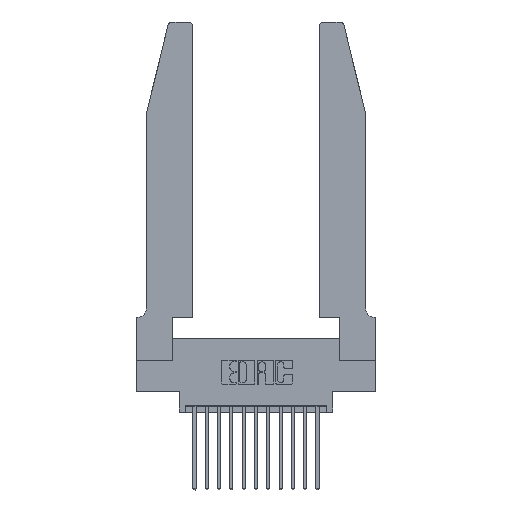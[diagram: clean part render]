
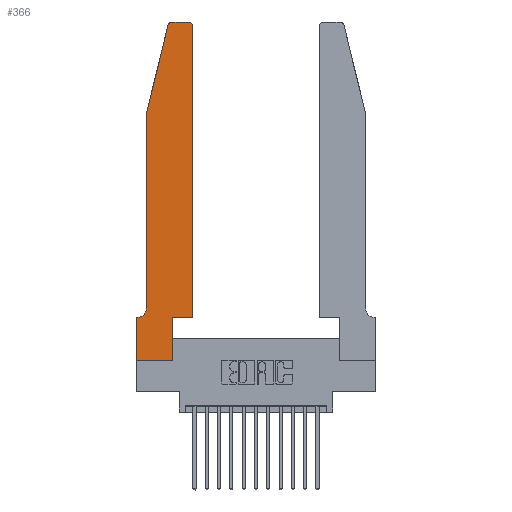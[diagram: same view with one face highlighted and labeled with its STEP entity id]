
A CAD part, top view. The second image highlights one B-rep face of the part: STEP entity #366.
In plain terms, the highlighted planar face has unit normal (0, 0, 1).
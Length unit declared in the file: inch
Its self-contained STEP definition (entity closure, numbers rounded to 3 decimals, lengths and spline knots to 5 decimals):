
#36 = DIRECTION ( 'NONE',  ( 1., 0., 0. ) ) ;
#366 = ADVANCED_FACE ( 'NONE', ( #13442 ), #1241, .T. ) ;
#414 = ORIENTED_EDGE ( 'NONE', *, *, #12444, .T. ) ;
#438 = LINE ( 'NONE', #11893, #1290 ) ;
#743 = EDGE_CURVE ( 'NONE', #1379, #2221, #4487, .T. ) ;
#882 = DIRECTION ( 'NONE',  ( 0., 0., -1. ) ) ;
#923 = CARTESIAN_POINT ( 'NONE',  ( 0.0055, 0.35, 0.37 ) ) ;
#1241 = PLANE ( 'NONE',  #9809 ) ;
#1269 = DIRECTION ( 'NONE',  ( 1., 0., 0. ) ) ;
#1290 = VECTOR ( 'NONE', #7604, 39.37008 ) ;
#1333 = CARTESIAN_POINT ( 'NONE',  ( 0.2865, 0.35, 0.37 ) ) ;
#1379 = VERTEX_POINT ( 'NONE', #923 ) ;
#1514 = VECTOR ( 'NONE', #6909, 39.37008 ) ;
#1750 = VECTOR ( 'NONE', #2633, 39.37008 ) ;
#1841 = VERTEX_POINT ( 'NONE', #9988 ) ;
#1915 = VECTOR ( 'NONE', #12813, 39.37008 ) ;
#2221 = VERTEX_POINT ( 'NONE', #14947 ) ;
#2362 = CARTESIAN_POINT ( 'NONE',  ( 0.2605, 2.75, 0.37 ) ) ;
#2605 = DIRECTION ( 'NONE',  ( 1., 0., 0. ) ) ;
#2621 = CARTESIAN_POINT ( 'NONE',  ( 0.2865, 0., 0.37 ) ) ;
#2633 = DIRECTION ( 'NONE',  ( 0., 1., 0. ) ) ;
#2759 = ORIENTED_EDGE ( 'NONE', *, *, #6326, .T. ) ;
#2988 = AXIS2_PLACEMENT_3D ( 'NONE', #9457, #16083, #1269 ) ;
#3045 = EDGE_CURVE ( 'NONE', #14107, #12969, #438, .T. ) ;
#3153 = DIRECTION ( 'NONE',  ( 0., -1., 0. ) ) ;
#3775 = VERTEX_POINT ( 'NONE', #7688 ) ;
#3949 = VERTEX_POINT ( 'NONE', #13862 ) ;
#4215 = CARTESIAN_POINT ( 'NONE',  ( 0.4205, 2.72, 0.37 ) ) ;
#4487 = LINE ( 'NONE', #15504, #1915 ) ;
#4493 = LINE ( 'NONE', #12278, #10693 ) ;
#4571 = VECTOR ( 'NONE', #3153, 39.37008 ) ;
#4719 = CARTESIAN_POINT ( 'NONE',  ( 0., 0., 0.37 ) ) ;
#5234 = DIRECTION ( 'NONE',  ( 1., 0., 0. ) ) ;
#5677 = LINE ( 'NONE', #2362, #12082 ) ;
#5840 = ORIENTED_EDGE ( 'NONE', *, *, #16171, .T. ) ;
#6107 = DIRECTION ( 'NONE',  ( 1., 0., 0. ) ) ;
#6326 = EDGE_CURVE ( 'NONE', #3775, #12021, #15503, .T. ) ;
#6420 = CARTESIAN_POINT ( 'NONE',  ( 0.0755, 0.42, 0.37 ) ) ;
#6518 = EDGE_LOOP ( 'NONE', ( #13067, #2759, #12171, #9908, #8247, #12234, #15975, #414, #17233, #5840, #12207, #11344 ) ) ;
#6736 = DIRECTION ( 'NONE',  ( 0., 0., 1. ) ) ;
#6799 = LINE ( 'NONE', #4719, #15591 ) ;
#6909 = DIRECTION ( 'NONE',  ( 0., -1., 0. ) ) ;
#7012 = DIRECTION ( 'NONE',  ( 0., 0., 1. ) ) ;
#7041 = EDGE_CURVE ( 'NONE', #16022, #16143, #11839, .T. ) ;
#7582 = DIRECTION ( 'NONE',  ( -1., 0., 0. ) ) ;
#7604 = DIRECTION ( 'NONE',  ( 0., 1., 0. ) ) ;
#7688 = CARTESIAN_POINT ( 'NONE',  ( 0.284, 2.75, 0.37 ) ) ;
#7860 = CARTESIAN_POINT ( 'NONE',  ( 0.4505, 0.35, 0.37 ) ) ;
#8030 = CIRCLE ( 'NONE', #10823, 0.07 ) ;
#8247 = ORIENTED_EDGE ( 'NONE', *, *, #17487, .T. ) ;
#8528 = CARTESIAN_POINT ( 'NONE',  ( 0.4505, 2.72, 0.37 ) ) ;
#8887 = EDGE_CURVE ( 'NONE', #2221, #3949, #16049, .T. ) ;
#9457 = CARTESIAN_POINT ( 'NONE',  ( 0.284, 2.72, 0.37 ) ) ;
#9809 = AXIS2_PLACEMENT_3D ( 'NONE', #14852, #6736, #2605 ) ;
#9860 = CARTESIAN_POINT ( 'NONE',  ( 0.0755, 2., 0.37 ) ) ;
#9908 = ORIENTED_EDGE ( 'NONE', *, *, #7041, .T. ) ;
#9988 = CARTESIAN_POINT ( 'NONE',  ( 0.4205, 2.75, 0.37 ) ) ;
#10546 = EDGE_CURVE ( 'NONE', #15060, #11377, #10751, .T. ) ;
#10693 = VECTOR ( 'NONE', #13590, 39.37008 ) ;
#10751 = LINE ( 'NONE', #1333, #1750 ) ;
#10823 = AXIS2_PLACEMENT_3D ( 'NONE', #17265, #882, #7582 ) ;
#11344 = ORIENTED_EDGE ( 'NONE', *, *, #11554, .T. ) ;
#11377 = VERTEX_POINT ( 'NONE', #17323 ) ;
#11502 = EDGE_CURVE ( 'NONE', #12021, #16022, #4493, .T. ) ;
#11554 = EDGE_CURVE ( 'NONE', #12969, #1841, #16480, .T. ) ;
#11839 = LINE ( 'NONE', #9860, #4571 ) ;
#11893 = CARTESIAN_POINT ( 'NONE',  ( 0.4505, 0.35, 0.37 ) ) ;
#11928 = AXIS2_PLACEMENT_3D ( 'NONE', #4215, #7012, #36 ) ;
#12021 = VERTEX_POINT ( 'NONE', #13398 ) ;
#12082 = VECTOR ( 'NONE', #15931, 39.37008 ) ;
#12171 = ORIENTED_EDGE ( 'NONE', *, *, #11502, .T. ) ;
#12207 = ORIENTED_EDGE ( 'NONE', *, *, #3045, .T. ) ;
#12234 = ORIENTED_EDGE ( 'NONE', *, *, #743, .T. ) ;
#12278 = CARTESIAN_POINT ( 'NONE',  ( 0.0755, 2., 0.37 ) ) ;
#12444 = EDGE_CURVE ( 'NONE', #3949, #15060, #6799, .T. ) ;
#12813 = DIRECTION ( 'NONE',  ( -1., 0., 0. ) ) ;
#12969 = VERTEX_POINT ( 'NONE', #8528 ) ;
#13067 = ORIENTED_EDGE ( 'NONE', *, *, #17464, .T. ) ;
#13107 = CARTESIAN_POINT ( 'NONE',  ( 0.0755, 2., 0.37 ) ) ;
#13398 = CARTESIAN_POINT ( 'NONE',  ( 0.25487, 2.72718, 0.37 ) ) ;
#13442 = FACE_OUTER_BOUND ( 'NONE', #6518, .T. ) ;
#13590 = DIRECTION ( 'NONE',  ( -0.239, -0.971, 0. ) ) ;
#13862 = CARTESIAN_POINT ( 'NONE',  ( 0., 0., 0.37 ) ) ;
#14107 = VERTEX_POINT ( 'NONE', #15625 ) ;
#14797 = VECTOR ( 'NONE', #5234, 39.37008 ) ;
#14852 = CARTESIAN_POINT ( 'NONE',  ( 0., 0.35, 0.37 ) ) ;
#14947 = CARTESIAN_POINT ( 'NONE',  ( 0., 0.35, 0.37 ) ) ;
#15060 = VERTEX_POINT ( 'NONE', #2621 ) ;
#15232 = LINE ( 'NONE', #7860, #14797 ) ;
#15503 = CIRCLE ( 'NONE', #2988, 0.03 ) ;
#15504 = CARTESIAN_POINT ( 'NONE',  ( 0.0755, 0.35, 0.37 ) ) ;
#15591 = VECTOR ( 'NONE', #6107, 39.37008 ) ;
#15625 = CARTESIAN_POINT ( 'NONE',  ( 0.4505, 0.35, 0.37 ) ) ;
#15931 = DIRECTION ( 'NONE',  ( -1., 0., 0. ) ) ;
#15975 = ORIENTED_EDGE ( 'NONE', *, *, #8887, .T. ) ;
#16022 = VERTEX_POINT ( 'NONE', #13107 ) ;
#16049 = LINE ( 'NONE', #17689, #1514 ) ;
#16083 = DIRECTION ( 'NONE',  ( 0., 0., 1. ) ) ;
#16143 = VERTEX_POINT ( 'NONE', #6420 ) ;
#16171 = EDGE_CURVE ( 'NONE', #11377, #14107, #15232, .T. ) ;
#16480 = CIRCLE ( 'NONE', #11928, 0.03 ) ;
#17233 = ORIENTED_EDGE ( 'NONE', *, *, #10546, .T. ) ;
#17265 = CARTESIAN_POINT ( 'NONE',  ( 0.0055, 0.42, 0.37 ) ) ;
#17323 = CARTESIAN_POINT ( 'NONE',  ( 0.2865, 0.35, 0.37 ) ) ;
#17464 = EDGE_CURVE ( 'NONE', #1841, #3775, #5677, .T. ) ;
#17487 = EDGE_CURVE ( 'NONE', #16143, #1379, #8030, .T. ) ;
#17689 = CARTESIAN_POINT ( 'NONE',  ( 0., 0., 0.37 ) ) ;
